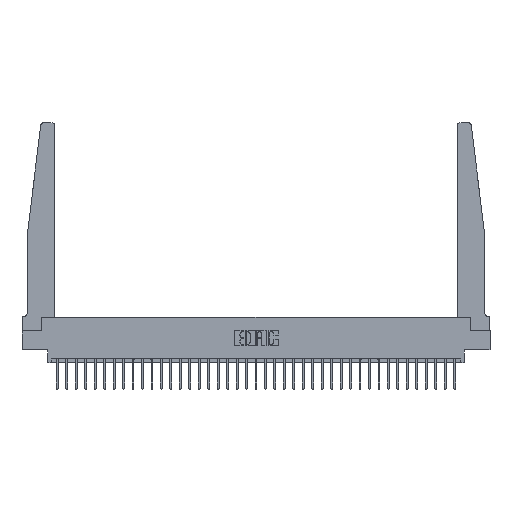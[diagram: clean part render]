
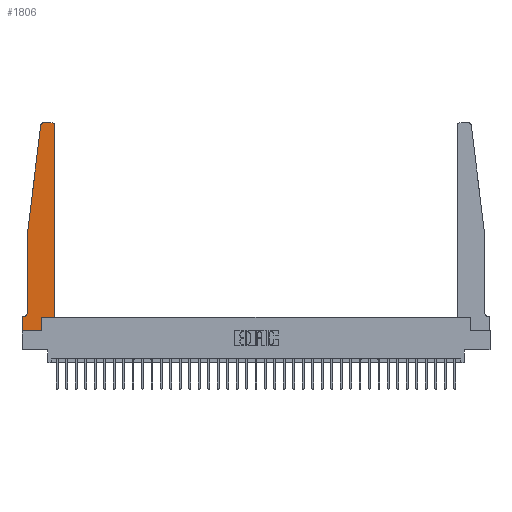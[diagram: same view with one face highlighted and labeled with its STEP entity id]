
A CAD part, top view. The second image highlights one B-rep face of the part: STEP entity #1806.
In plain terms, the highlighted planar face has unit normal (0, 0, 1).
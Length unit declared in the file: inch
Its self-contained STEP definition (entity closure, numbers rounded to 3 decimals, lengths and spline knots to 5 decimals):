
#106 = LINE ( 'NONE', #26131, #31495 ) ;
#786 = VERTEX_POINT ( 'NONE', #20579 ) ;
#1063 = DIRECTION ( 'NONE',  ( -1., 0., 0. ) ) ;
#1434 = CARTESIAN_POINT ( 'NONE',  ( 0., 0., 0.37 ) ) ;
#1806 = ADVANCED_FACE ( 'NONE', ( #24001 ), #17929, .T. ) ;
#2408 = ORIENTED_EDGE ( 'NONE', *, *, #12633, .T. ) ;
#2522 = CARTESIAN_POINT ( 'NONE',  ( 0.425, 0.18, 0.37 ) ) ;
#2528 = DIRECTION ( 'NONE',  ( 0., 1., 0. ) ) ;
#3436 = VECTOR ( 'NONE', #8634, 39.37008 ) ;
#3808 = VERTEX_POINT ( 'NONE', #31048 ) ;
#4779 = CARTESIAN_POINT ( 'NONE',  ( 0.425, 2.72, 0.37 ) ) ;
#6251 = ORIENTED_EDGE ( 'NONE', *, *, #24887, .T. ) ;
#6785 = CARTESIAN_POINT ( 'NONE',  ( 0.425, 0.18, 0.37 ) ) ;
#7007 = CARTESIAN_POINT ( 'NONE',  ( 0.065, 1.25, 0.37 ) ) ;
#7780 = CARTESIAN_POINT ( 'NONE',  ( 0.065, 0.2375, 0.37 ) ) ;
#8539 = CARTESIAN_POINT ( 'NONE',  ( 0.065, 1.25, 0.37 ) ) ;
#8634 = DIRECTION ( 'NONE',  ( -1., 0., 0. ) ) ;
#9082 = DIRECTION ( 'NONE',  ( 0., 0., 1. ) ) ;
#9314 = AXIS2_PLACEMENT_3D ( 'NONE', #12184, #29795, #14749 ) ;
#9340 = VERTEX_POINT ( 'NONE', #25262 ) ;
#9375 = AXIS2_PLACEMENT_3D ( 'NONE', #24273, #9082, #26821 ) ;
#9378 = CARTESIAN_POINT ( 'NONE',  ( 0., 0., 0.37 ) ) ;
#9636 = LINE ( 'NONE', #17919, #15644 ) ;
#9880 = AXIS2_PLACEMENT_3D ( 'NONE', #29372, #14330, #31909 ) ;
#10108 = CARTESIAN_POINT ( 'NONE',  ( 0.065, 1.25, 0.37 ) ) ;
#10327 = DIRECTION ( 'NONE',  ( 0., 0., 1. ) ) ;
#10364 = VERTEX_POINT ( 'NONE', #19204 ) ;
#10449 = EDGE_CURVE ( 'NONE', #11115, #3808, #16421, .T. ) ;
#10911 = LINE ( 'NONE', #12599, #31025 ) ;
#11102 = LINE ( 'NONE', #26380, #3436 ) ;
#11115 = VERTEX_POINT ( 'NONE', #4779 ) ;
#11184 = CARTESIAN_POINT ( 'NONE',  ( 0.2605, 0., 0.37 ) ) ;
#11606 = VERTEX_POINT ( 'NONE', #11846 ) ;
#11657 = VERTEX_POINT ( 'NONE', #9378 ) ;
#11846 = CARTESIAN_POINT ( 'NONE',  ( 0., 0.1875, 0.37 ) ) ;
#12184 = CARTESIAN_POINT ( 'NONE',  ( 0.395, 2.72, 0.37 ) ) ;
#12228 = ORIENTED_EDGE ( 'NONE', *, *, #22321, .T. ) ;
#12599 = CARTESIAN_POINT ( 'NONE',  ( 0., 0., 0.37 ) ) ;
#12633 = EDGE_CURVE ( 'NONE', #786, #9340, #18268, .T. ) ;
#12698 = DIRECTION ( 'NONE',  ( 0., -1., 0. ) ) ;
#12885 = ORIENTED_EDGE ( 'NONE', *, *, #20368, .T. ) ;
#13323 = LINE ( 'NONE', #1434, #25924 ) ;
#13332 = VERTEX_POINT ( 'NONE', #6785 ) ;
#13799 = VECTOR ( 'NONE', #26281, 39.37008 ) ;
#14025 = CARTESIAN_POINT ( 'NONE',  ( 0.065, 0.1875, 0.37 ) ) ;
#14031 = EDGE_CURVE ( 'NONE', #21070, #24267, #106, .T. ) ;
#14205 = CIRCLE ( 'NONE', #9880, 0.05 ) ;
#14330 = DIRECTION ( 'NONE',  ( 0., 0., -1. ) ) ;
#14501 = ORIENTED_EDGE ( 'NONE', *, *, #31730, .T. ) ;
#14749 = DIRECTION ( 'NONE',  ( 1., 0., 0. ) ) ;
#15644 = VECTOR ( 'NONE', #2528, 39.37008 ) ;
#16209 = EDGE_CURVE ( 'NONE', #29709, #10364, #14205, .T. ) ;
#16421 = CIRCLE ( 'NONE', #9314, 0.03 ) ;
#16551 = ORIENTED_EDGE ( 'NONE', *, *, #10449, .T. ) ;
#17287 = EDGE_CURVE ( 'NONE', #11657, #21070, #10911, .T. ) ;
#17590 = VECTOR ( 'NONE', #1063, 39.37008 ) ;
#17622 = EDGE_CURVE ( 'NONE', #11606, #11657, #13323, .T. ) ;
#17654 = EDGE_LOOP ( 'NONE', ( #12885, #2408, #12228, #6251, #29583, #18677, #28695, #30574, #21850, #19136, #14501, #16551 ) ) ;
#17919 = CARTESIAN_POINT ( 'NONE',  ( 0.425, 0.18, 0.37 ) ) ;
#17929 = PLANE ( 'NONE',  #25106 ) ;
#18268 = CIRCLE ( 'NONE', #9375, 0.03 ) ;
#18365 = VERTEX_POINT ( 'NONE', #7007 ) ;
#18587 = DIRECTION ( 'NONE',  ( 0., 1., 0. ) ) ;
#18677 = ORIENTED_EDGE ( 'NONE', *, *, #23139, .T. ) ;
#19136 = ORIENTED_EDGE ( 'NONE', *, *, #28980, .T. ) ;
#19204 = CARTESIAN_POINT ( 'NONE',  ( 0.015, 0.1875, 0.37 ) ) ;
#19757 = LINE ( 'NONE', #8539, #13799 ) ;
#19854 = VECTOR ( 'NONE', #12698, 39.37008 ) ;
#20368 = EDGE_CURVE ( 'NONE', #3808, #786, #11102, .T. ) ;
#20424 = DIRECTION ( 'NONE',  ( 1., 0., 0. ) ) ;
#20579 = CARTESIAN_POINT ( 'NONE',  ( 0.27653, 2.75, 0.37 ) ) ;
#21070 = VERTEX_POINT ( 'NONE', #11184 ) ;
#21850 = ORIENTED_EDGE ( 'NONE', *, *, #14031, .T. ) ;
#22321 = EDGE_CURVE ( 'NONE', #9340, #18365, #19757, .T. ) ;
#22349 = VECTOR ( 'NONE', #20424, 39.37008 ) ;
#22954 = CARTESIAN_POINT ( 'NONE',  ( 0., 0.1875, 0.37 ) ) ;
#23136 = LINE ( 'NONE', #2522, #22349 ) ;
#23139 = EDGE_CURVE ( 'NONE', #10364, #11606, #23461, .T. ) ;
#23203 = CARTESIAN_POINT ( 'NONE',  ( 0.2605, 0.18, 0.37 ) ) ;
#23461 = LINE ( 'NONE', #14025, #17590 ) ;
#24001 = FACE_OUTER_BOUND ( 'NONE', #17654, .T. ) ;
#24267 = VERTEX_POINT ( 'NONE', #23203 ) ;
#24273 = CARTESIAN_POINT ( 'NONE',  ( 0.27653, 2.72, 0.37 ) ) ;
#24384 = DIRECTION ( 'NONE',  ( 0., -1., 0. ) ) ;
#24887 = EDGE_CURVE ( 'NONE', #18365, #29709, #26507, .T. ) ;
#25106 = AXIS2_PLACEMENT_3D ( 'NONE', #22954, #10327, #28008 ) ;
#25262 = CARTESIAN_POINT ( 'NONE',  ( 0.24675, 2.72367, 0.37 ) ) ;
#25924 = VECTOR ( 'NONE', #24384, 39.37008 ) ;
#26131 = CARTESIAN_POINT ( 'NONE',  ( 0.2605, 0.18, 0.37 ) ) ;
#26281 = DIRECTION ( 'NONE',  ( -0.122, -0.992, 0. ) ) ;
#26380 = CARTESIAN_POINT ( 'NONE',  ( 0.25, 2.75, 0.37 ) ) ;
#26507 = LINE ( 'NONE', #10108, #19854 ) ;
#26821 = DIRECTION ( 'NONE',  ( 1., 0., 0. ) ) ;
#28008 = DIRECTION ( 'NONE',  ( 1., 0., 0. ) ) ;
#28695 = ORIENTED_EDGE ( 'NONE', *, *, #17622, .T. ) ;
#28980 = EDGE_CURVE ( 'NONE', #24267, #13332, #23136, .T. ) ;
#29372 = CARTESIAN_POINT ( 'NONE',  ( 0.015, 0.2375, 0.37 ) ) ;
#29583 = ORIENTED_EDGE ( 'NONE', *, *, #16209, .T. ) ;
#29709 = VERTEX_POINT ( 'NONE', #7780 ) ;
#29795 = DIRECTION ( 'NONE',  ( 0., 0., 1. ) ) ;
#30574 = ORIENTED_EDGE ( 'NONE', *, *, #17287, .T. ) ;
#31025 = VECTOR ( 'NONE', #32713, 39.37008 ) ;
#31048 = CARTESIAN_POINT ( 'NONE',  ( 0.395, 2.75, 0.37 ) ) ;
#31495 = VECTOR ( 'NONE', #18587, 39.37008 ) ;
#31730 = EDGE_CURVE ( 'NONE', #13332, #11115, #9636, .T. ) ;
#31909 = DIRECTION ( 'NONE',  ( -1., 0., 0. ) ) ;
#32713 = DIRECTION ( 'NONE',  ( 1., 0., 0. ) ) ;
